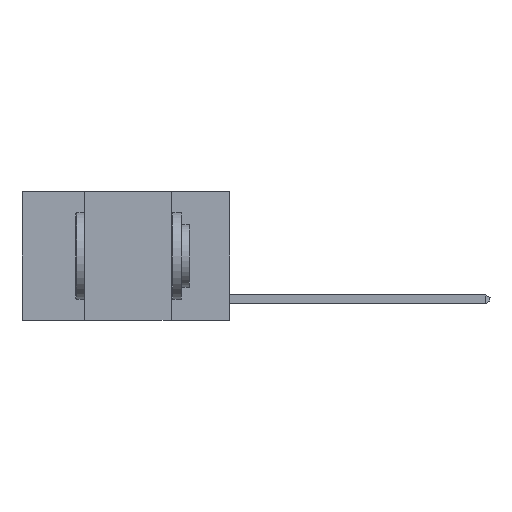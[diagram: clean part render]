
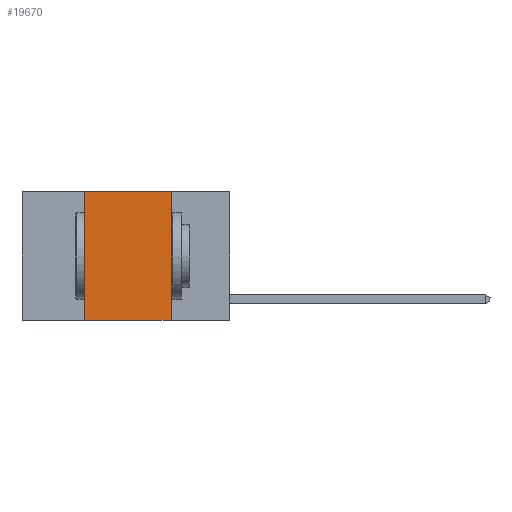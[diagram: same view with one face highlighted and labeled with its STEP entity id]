
A CAD part, left-side view. The second image highlights one B-rep face of the part: STEP entity #19670.
In plain terms, the highlighted planar face has unit normal (-1, 0, 0).
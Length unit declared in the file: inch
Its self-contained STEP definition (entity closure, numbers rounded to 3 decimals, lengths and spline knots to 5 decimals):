
#58 = EDGE_CURVE ( 'NONE', #16152, #14608, #1826, .T. ) ;
#250 = DIRECTION ( 'NONE',  ( 1., 0., 0. ) ) ;
#472 = ORIENTED_EDGE ( 'NONE', *, *, #58, .T. ) ;
#1749 = DIRECTION ( 'NONE',  ( 0., 0., 1. ) ) ;
#1826 = LINE ( 'NONE', #11711, #16848 ) ;
#1828 = CARTESIAN_POINT ( 'NONE',  ( 0., 0.17, 0. ) ) ;
#1867 = PLANE ( 'NONE',  #12971 ) ;
#2182 = EDGE_CURVE ( 'NONE', #16152, #24920, #15498, .T. ) ;
#2482 = VECTOR ( 'NONE', #25391, 39.37008 ) ;
#3713 = LINE ( 'NONE', #1828, #20737 ) ;
#5487 = ORIENTED_EDGE ( 'NONE', *, *, #23110, .F. ) ;
#5534 = DIRECTION ( 'NONE',  ( 0., 0., -1. ) ) ;
#5577 = CARTESIAN_POINT ( 'NONE',  ( 0., 0.17, -0.37 ) ) ;
#6475 = ORIENTED_EDGE ( 'NONE', *, *, #2182, .F. ) ;
#8891 = CARTESIAN_POINT ( 'NONE',  ( 0., 0.42, -0.37 ) ) ;
#10463 = VECTOR ( 'NONE', #1749, 39.37008 ) ;
#11711 = CARTESIAN_POINT ( 'NONE',  ( 0., 0.6, -0.37 ) ) ;
#12971 = AXIS2_PLACEMENT_3D ( 'NONE', #21641, #250, #5534 ) ;
#13429 = LINE ( 'NONE', #17284, #2482 ) ;
#13764 = CARTESIAN_POINT ( 'NONE',  ( 0., 0.42, 0. ) ) ;
#13849 = DIRECTION ( 'NONE',  ( 0., 0., -1. ) ) ;
#14608 = VERTEX_POINT ( 'NONE', #5577 ) ;
#15199 = VERTEX_POINT ( 'NONE', #23500 ) ;
#15498 = LINE ( 'NONE', #13764, #10463 ) ;
#16152 = VERTEX_POINT ( 'NONE', #8891 ) ;
#16848 = VECTOR ( 'NONE', #19841, 39.37008 ) ;
#17284 = CARTESIAN_POINT ( 'NONE',  ( 0., 0.6, 0. ) ) ;
#19670 = ADVANCED_FACE ( 'NONE', ( #22266 ), #1867, .F. ) ;
#19841 = DIRECTION ( 'NONE',  ( 0., -1., 0. ) ) ;
#20380 = EDGE_LOOP ( 'NONE', ( #5487, #22241, #6475, #472 ) ) ;
#20737 = VECTOR ( 'NONE', #13849, 39.37008 ) ;
#21641 = CARTESIAN_POINT ( 'NONE',  ( 0., 0.6, 0. ) ) ;
#22241 = ORIENTED_EDGE ( 'NONE', *, *, #26097, .F. ) ;
#22266 = FACE_OUTER_BOUND ( 'NONE', #20380, .T. ) ;
#23110 = EDGE_CURVE ( 'NONE', #15199, #14608, #3713, .T. ) ;
#23500 = CARTESIAN_POINT ( 'NONE',  ( 0., 0.17, 0. ) ) ;
#23681 = CARTESIAN_POINT ( 'NONE',  ( 0., 0.42, 0. ) ) ;
#24920 = VERTEX_POINT ( 'NONE', #23681 ) ;
#25391 = DIRECTION ( 'NONE',  ( 0., -1., 0. ) ) ;
#26097 = EDGE_CURVE ( 'NONE', #24920, #15199, #13429, .T. ) ;
